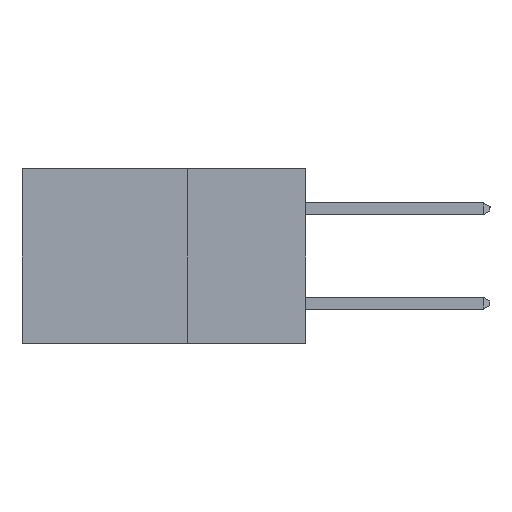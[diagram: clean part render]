
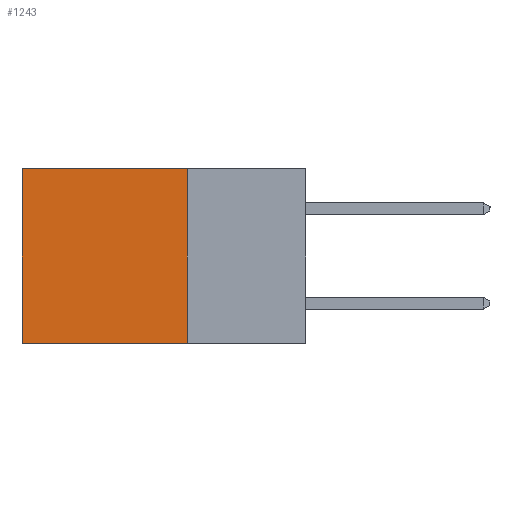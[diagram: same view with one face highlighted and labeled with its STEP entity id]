
A CAD part, left-side view. The second image highlights one B-rep face of the part: STEP entity #1243.
In plain terms, the highlighted planar face has unit normal (-1, 0, 0).
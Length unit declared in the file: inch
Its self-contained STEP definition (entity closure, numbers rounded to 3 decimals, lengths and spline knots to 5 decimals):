
#287 = ORIENTED_EDGE ( 'NONE', *, *, #8138, .T. ) ;
#980 = LINE ( 'NONE', #4214, #3058 ) ;
#995 = DIRECTION ( 'NONE',  ( 0., 0., -1. ) ) ;
#1001 = CARTESIAN_POINT ( 'NONE',  ( 0.2615, 0.25, -0.37 ) ) ;
#1243 = ADVANCED_FACE ( 'NONE', ( #2536 ), #7300, .F. ) ;
#1247 = CARTESIAN_POINT ( 'NONE',  ( 0.2615, 0.6, -0.37 ) ) ;
#1818 = EDGE_CURVE ( 'NONE', #8727, #7666, #980, .T. ) ;
#2536 = FACE_OUTER_BOUND ( 'NONE', #9231, .T. ) ;
#2694 = DIRECTION ( 'NONE',  ( 0., 0., -1. ) ) ;
#2799 = CARTESIAN_POINT ( 'NONE',  ( 0.2615, 0.6, -0.37 ) ) ;
#3058 = VECTOR ( 'NONE', #4112, 39.37008 ) ;
#3359 = DIRECTION ( 'NONE',  ( 0., 0., -1. ) ) ;
#3503 = LINE ( 'NONE', #9970, #7097 ) ;
#3589 = LINE ( 'NONE', #1247, #7518 ) ;
#3661 = VERTEX_POINT ( 'NONE', #7203 ) ;
#3731 = CARTESIAN_POINT ( 'NONE',  ( 0.2615, 0.25, -0.37 ) ) ;
#4112 = DIRECTION ( 'NONE',  ( 0., 1., 0. ) ) ;
#4214 = CARTESIAN_POINT ( 'NONE',  ( 0.2615, 0.25, -0.37 ) ) ;
#4693 = AXIS2_PLACEMENT_3D ( 'NONE', #8768, #8717, #995 ) ;
#4700 = CARTESIAN_POINT ( 'NONE',  ( 0.2615, 0.6, 0. ) ) ;
#5554 = EDGE_CURVE ( 'NONE', #3661, #9178, #3503, .T. ) ;
#5725 = LINE ( 'NONE', #1001, #7352 ) ;
#6315 = ORIENTED_EDGE ( 'NONE', *, *, #5554, .T. ) ;
#6327 = ORIENTED_EDGE ( 'NONE', *, *, #7899, .F. ) ;
#7097 = VECTOR ( 'NONE', #7897, 39.37008 ) ;
#7203 = CARTESIAN_POINT ( 'NONE',  ( 0.2615, 0.25, 0. ) ) ;
#7300 = PLANE ( 'NONE',  #4693 ) ;
#7352 = VECTOR ( 'NONE', #3359, 39.37008 ) ;
#7518 = VECTOR ( 'NONE', #2694, 39.37008 ) ;
#7666 = VERTEX_POINT ( 'NONE', #2799 ) ;
#7897 = DIRECTION ( 'NONE',  ( 0., 1., 0. ) ) ;
#7899 = EDGE_CURVE ( 'NONE', #3661, #8727, #5725, .T. ) ;
#8138 = EDGE_CURVE ( 'NONE', #9178, #7666, #3589, .T. ) ;
#8221 = ORIENTED_EDGE ( 'NONE', *, *, #1818, .F. ) ;
#8717 = DIRECTION ( 'NONE',  ( 1., 0., 0. ) ) ;
#8727 = VERTEX_POINT ( 'NONE', #3731 ) ;
#8768 = CARTESIAN_POINT ( 'NONE',  ( 0.2615, 0.25, -0.37 ) ) ;
#9178 = VERTEX_POINT ( 'NONE', #4700 ) ;
#9231 = EDGE_LOOP ( 'NONE', ( #287, #8221, #6327, #6315 ) ) ;
#9970 = CARTESIAN_POINT ( 'NONE',  ( 0.2615, 0.25, 0. ) ) ;
